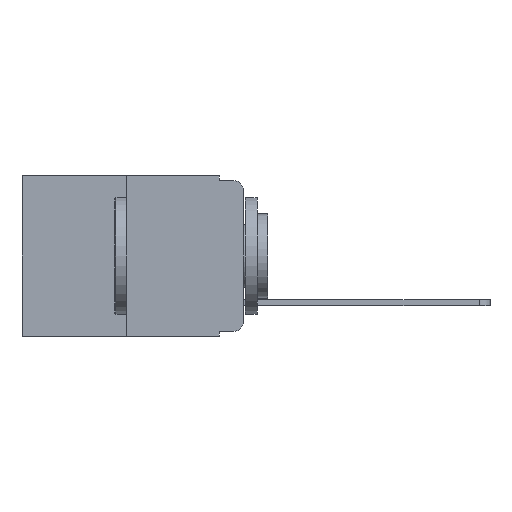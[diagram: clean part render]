
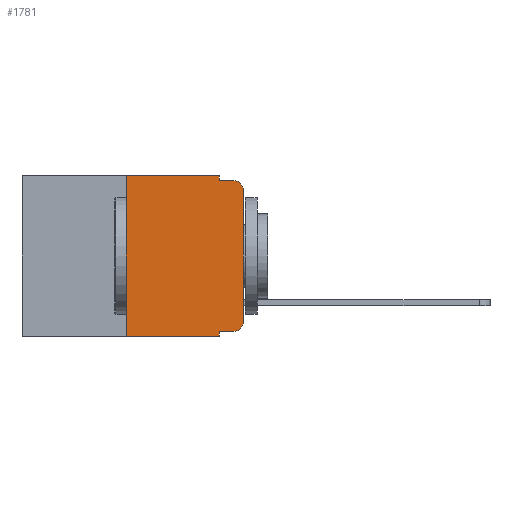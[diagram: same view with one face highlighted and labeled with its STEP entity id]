
A CAD part, left-side view. The second image highlights one B-rep face of the part: STEP entity #1781.
In plain terms, the highlighted planar face has unit normal (-1, 0, 0).
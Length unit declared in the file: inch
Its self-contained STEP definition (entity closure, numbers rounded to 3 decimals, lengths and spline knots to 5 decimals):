
#485 = DIRECTION ( 'NONE',  ( 0., 0., -1. ) ) ;
#578 = PLANE ( 'NONE',  #5418 ) ;
#751 = VERTEX_POINT ( 'NONE', #3364 ) ;
#964 = CARTESIAN_POINT ( 'NONE',  ( 0., 0.25, 0. ) ) ;
#1220 = CARTESIAN_POINT ( 'NONE',  ( 0., 0., -0.03 ) ) ;
#1459 = CIRCLE ( 'NONE', #3845, 0.02 ) ;
#1732 = CARTESIAN_POINT ( 'NONE',  ( 0., 0.02, -0.333 ) ) ;
#1781 = ADVANCED_FACE ( 'NONE', ( #13097 ), #578, .F. ) ;
#2038 = EDGE_CURVE ( 'NONE', #751, #12787, #12908, .T. ) ;
#2071 = LINE ( 'NONE', #14001, #11216 ) ;
#2223 = VECTOR ( 'NONE', #12814, 39.37008 ) ;
#2481 = CARTESIAN_POINT ( 'NONE',  ( 0., 0.051, -0.343 ) ) ;
#2600 = VECTOR ( 'NONE', #485, 39.37008 ) ;
#2844 = VERTEX_POINT ( 'NONE', #4175 ) ;
#3136 = ORIENTED_EDGE ( 'NONE', *, *, #7528, .F. ) ;
#3257 = DIRECTION ( 'NONE',  ( 0., 0., -1. ) ) ;
#3303 = EDGE_CURVE ( 'NONE', #10425, #14287, #1459, .T. ) ;
#3364 = CARTESIAN_POINT ( 'NONE',  ( 0., 0.25, 0. ) ) ;
#3727 = VECTOR ( 'NONE', #8913, 39.37008 ) ;
#3845 = AXIS2_PLACEMENT_3D ( 'NONE', #11636, #4988, #4952 ) ;
#3921 = VECTOR ( 'NONE', #14765, 39.37008 ) ;
#3957 = ORIENTED_EDGE ( 'NONE', *, *, #11302, .T. ) ;
#4167 = EDGE_CURVE ( 'NONE', #10235, #10425, #8945, .T. ) ;
#4175 = CARTESIAN_POINT ( 'NONE',  ( 0., 0.051, -0.01 ) ) ;
#4331 = ORIENTED_EDGE ( 'NONE', *, *, #4167, .T. ) ;
#4821 = VECTOR ( 'NONE', #6104, 39.37008 ) ;
#4856 = CARTESIAN_POINT ( 'NONE',  ( 0., 0.02, -0.03 ) ) ;
#4871 = DIRECTION ( 'NONE',  ( 0., 0., 1. ) ) ;
#4952 = DIRECTION ( 'NONE',  ( 0., 0., -1. ) ) ;
#4988 = DIRECTION ( 'NONE',  ( -1., 0., 0. ) ) ;
#5029 = EDGE_CURVE ( 'NONE', #10235, #11327, #9297, .T. ) ;
#5418 = AXIS2_PLACEMENT_3D ( 'NONE', #9224, #5875, #3257 ) ;
#5863 = EDGE_CURVE ( 'NONE', #11684, #751, #9039, .T. ) ;
#5875 = DIRECTION ( 'NONE',  ( 1., 0., 0. ) ) ;
#6104 = DIRECTION ( 'NONE',  ( 0., -1., 0. ) ) ;
#6117 = DIRECTION ( 'NONE',  ( 0., 0., -1. ) ) ;
#6307 = AXIS2_PLACEMENT_3D ( 'NONE', #4856, #13181, #6117 ) ;
#6679 = EDGE_CURVE ( 'NONE', #12787, #2844, #6829, .T. ) ;
#6829 = LINE ( 'NONE', #10328, #3921 ) ;
#6879 = ORIENTED_EDGE ( 'NONE', *, *, #2038, .F. ) ;
#7528 = EDGE_CURVE ( 'NONE', #2844, #11698, #2071, .T. ) ;
#8079 = ORIENTED_EDGE ( 'NONE', *, *, #3303, .T. ) ;
#8393 = EDGE_CURVE ( 'NONE', #14219, #11698, #11376, .T. ) ;
#8631 = CARTESIAN_POINT ( 'NONE',  ( 0., 0.25, -0.343 ) ) ;
#8893 = CARTESIAN_POINT ( 'NONE',  ( 0., 0., -0.313 ) ) ;
#8913 = DIRECTION ( 'NONE',  ( 0., -1., 0. ) ) ;
#8945 = LINE ( 'NONE', #14671, #4821 ) ;
#9039 = LINE ( 'NONE', #964, #14713 ) ;
#9209 = EDGE_CURVE ( 'NONE', #14287, #14219, #11988, .T. ) ;
#9224 = CARTESIAN_POINT ( 'NONE',  ( 0., 0.473, 0. ) ) ;
#9297 = LINE ( 'NONE', #13253, #2600 ) ;
#9405 = EDGE_LOOP ( 'NONE', ( #15063, #12436, #3136, #12770, #6879, #10191, #3957, #13490, #4331, #8079 ) ) ;
#10054 = CARTESIAN_POINT ( 'NONE',  ( 0., 0.473, 0. ) ) ;
#10191 = ORIENTED_EDGE ( 'NONE', *, *, #5863, .F. ) ;
#10235 = VERTEX_POINT ( 'NONE', #14630 ) ;
#10328 = CARTESIAN_POINT ( 'NONE',  ( 0., 0.051, 0. ) ) ;
#10425 = VERTEX_POINT ( 'NONE', #1732 ) ;
#10564 = VECTOR ( 'NONE', #13314, 39.37008 ) ;
#11216 = VECTOR ( 'NONE', #15124, 39.37008 ) ;
#11302 = EDGE_CURVE ( 'NONE', #11684, #11327, #14215, .T. ) ;
#11327 = VERTEX_POINT ( 'NONE', #2481 ) ;
#11376 = CIRCLE ( 'NONE', #6307, 0.02 ) ;
#11636 = CARTESIAN_POINT ( 'NONE',  ( 0., 0.02, -0.313 ) ) ;
#11684 = VERTEX_POINT ( 'NONE', #8631 ) ;
#11698 = VERTEX_POINT ( 'NONE', #12109 ) ;
#11734 = CARTESIAN_POINT ( 'NONE',  ( 0., 0., 0. ) ) ;
#11988 = LINE ( 'NONE', #11734, #2223 ) ;
#12109 = CARTESIAN_POINT ( 'NONE',  ( 0., 0.02, -0.01 ) ) ;
#12176 = CARTESIAN_POINT ( 'NONE',  ( 0., 0.051, 0. ) ) ;
#12194 = CARTESIAN_POINT ( 'NONE',  ( 0., 0.473, -0.343 ) ) ;
#12436 = ORIENTED_EDGE ( 'NONE', *, *, #8393, .T. ) ;
#12770 = ORIENTED_EDGE ( 'NONE', *, *, #6679, .F. ) ;
#12787 = VERTEX_POINT ( 'NONE', #12176 ) ;
#12814 = DIRECTION ( 'NONE',  ( 0., 0., 1. ) ) ;
#12908 = LINE ( 'NONE', #10054, #3727 ) ;
#13097 = FACE_OUTER_BOUND ( 'NONE', #9405, .T. ) ;
#13181 = DIRECTION ( 'NONE',  ( -1., 0., 0. ) ) ;
#13253 = CARTESIAN_POINT ( 'NONE',  ( 0., 0.051, 0. ) ) ;
#13314 = DIRECTION ( 'NONE',  ( 0., -1., 0. ) ) ;
#13490 = ORIENTED_EDGE ( 'NONE', *, *, #5029, .F. ) ;
#14001 = CARTESIAN_POINT ( 'NONE',  ( 0., 0.051, -0.01 ) ) ;
#14215 = LINE ( 'NONE', #12194, #10564 ) ;
#14219 = VERTEX_POINT ( 'NONE', #1220 ) ;
#14287 = VERTEX_POINT ( 'NONE', #8893 ) ;
#14630 = CARTESIAN_POINT ( 'NONE',  ( 0., 0.051, -0.333 ) ) ;
#14671 = CARTESIAN_POINT ( 'NONE',  ( 0., 0.051, -0.333 ) ) ;
#14713 = VECTOR ( 'NONE', #4871, 39.37008 ) ;
#14765 = DIRECTION ( 'NONE',  ( 0., 0., -1. ) ) ;
#15063 = ORIENTED_EDGE ( 'NONE', *, *, #9209, .T. ) ;
#15124 = DIRECTION ( 'NONE',  ( 0., -1., 0. ) ) ;
